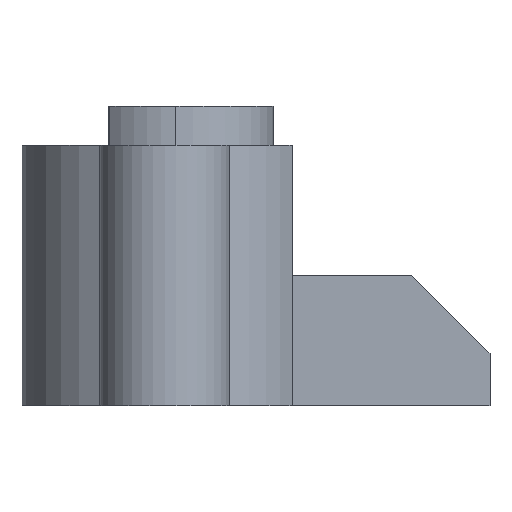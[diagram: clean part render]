
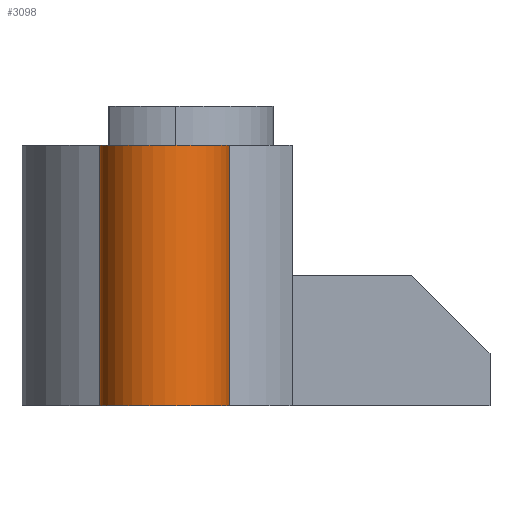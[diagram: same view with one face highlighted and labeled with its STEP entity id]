
A CAD part, left-side view. The second image highlights one B-rep face of the part: STEP entity #3098.
In plain terms, the highlighted cylindrical face has radius 2.5 mm (diameter 5 mm), a partial arc.
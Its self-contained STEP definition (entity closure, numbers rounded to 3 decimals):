
#317 = DIRECTION ( 'NONE',  ( 0., 0., -1. ) ) ;
#380 = DIRECTION ( 'NONE',  ( 1., 0., 0. ) ) ;
#486 = VERTEX_POINT ( 'NONE', #1484 ) ;
#492 = AXIS2_PLACEMENT_3D ( 'NONE', #3123, #860, #3489 ) ;
#551 = EDGE_LOOP ( 'NONE', ( #3142, #3268, #4004, #4124 ) ) ;
#560 = AXIS2_PLACEMENT_3D ( 'NONE', #3391, #1509, #380 ) ;
#751 = AXIS2_PLACEMENT_3D ( 'NONE', #1472, #4086, #1846 ) ;
#860 = DIRECTION ( 'NONE',  ( 0., 0., 1. ) ) ;
#1212 = CIRCLE ( 'NONE', #492, 2.5 ) ;
#1253 = VECTOR ( 'NONE', #317, 1000. ) ;
#1317 = DIRECTION ( 'NONE',  ( 0., 0., -1. ) ) ;
#1472 = CARTESIAN_POINT ( 'NONE',  ( -29.351, 23.292, 10. ) ) ;
#1484 = CARTESIAN_POINT ( 'NONE',  ( -29.351, 20.792, 10. ) ) ;
#1491 = FACE_OUTER_BOUND ( 'NONE', #551, .T. ) ;
#1509 = DIRECTION ( 'NONE',  ( 0., 0., 1. ) ) ;
#1719 = CARTESIAN_POINT ( 'NONE',  ( -29.351, 20.792, 10. ) ) ;
#1846 = DIRECTION ( 'NONE',  ( 1., 0., 0. ) ) ;
#2071 = VERTEX_POINT ( 'NONE', #4044 ) ;
#2269 = LINE ( 'NONE', #3630, #1253 ) ;
#2565 = EDGE_CURVE ( 'NONE', #3752, #2071, #2269, .T. ) ;
#3098 = ADVANCED_FACE ( 'NONE', ( #1491 ), #4353, .T. ) ;
#3123 = CARTESIAN_POINT ( 'NONE',  ( -29.351, 23.292, 0. ) ) ;
#3142 = ORIENTED_EDGE ( 'NONE', *, *, #3775, .T. ) ;
#3268 = ORIENTED_EDGE ( 'NONE', *, *, #4465, .F. ) ;
#3391 = CARTESIAN_POINT ( 'NONE',  ( -29.351, 23.292, 0. ) ) ;
#3451 = VECTOR ( 'NONE', #1317, 1000. ) ;
#3489 = DIRECTION ( 'NONE',  ( 1., 0., 0. ) ) ;
#3531 = VERTEX_POINT ( 'NONE', #4685 ) ;
#3630 = CARTESIAN_POINT ( 'NONE',  ( -29.351, 25.792, 10. ) ) ;
#3752 = VERTEX_POINT ( 'NONE', #3792 ) ;
#3775 = EDGE_CURVE ( 'NONE', #2071, #3531, #1212, .T. ) ;
#3792 = CARTESIAN_POINT ( 'NONE',  ( -29.351, 25.792, 10. ) ) ;
#4004 = ORIENTED_EDGE ( 'NONE', *, *, #4580, .F. ) ;
#4044 = CARTESIAN_POINT ( 'NONE',  ( -29.351, 25.792, 0. ) ) ;
#4086 = DIRECTION ( 'NONE',  ( 0., 0., 1. ) ) ;
#4091 = CIRCLE ( 'NONE', #751, 2.5 ) ;
#4124 = ORIENTED_EDGE ( 'NONE', *, *, #2565, .T. ) ;
#4353 = CYLINDRICAL_SURFACE ( 'NONE', #560, 2.5 ) ;
#4441 = LINE ( 'NONE', #1719, #3451 ) ;
#4465 = EDGE_CURVE ( 'NONE', #486, #3531, #4441, .T. ) ;
#4580 = EDGE_CURVE ( 'NONE', #3752, #486, #4091, .T. ) ;
#4685 = CARTESIAN_POINT ( 'NONE',  ( -29.351, 20.792, 0. ) ) ;
